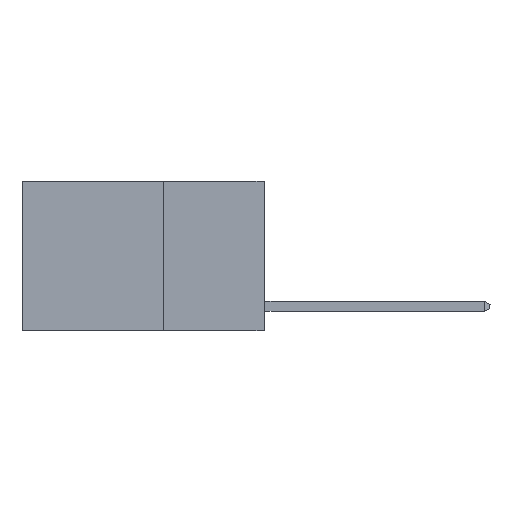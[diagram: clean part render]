
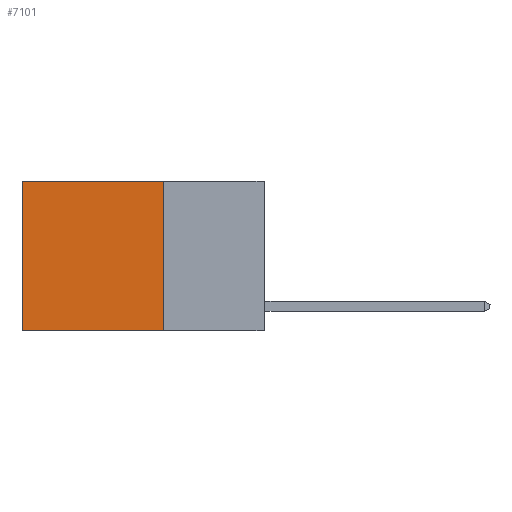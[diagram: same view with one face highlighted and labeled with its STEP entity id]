
A CAD part, left-side view. The second image highlights one B-rep face of the part: STEP entity #7101.
In plain terms, the highlighted planar face has unit normal (-1, 0, 0).
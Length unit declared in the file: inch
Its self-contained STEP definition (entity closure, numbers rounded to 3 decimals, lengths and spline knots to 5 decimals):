
#407 = EDGE_CURVE ( 'NONE', #5967, #1259, #1704, .T. ) ;
#1152 = CARTESIAN_POINT ( 'NONE',  ( 0.2625, 0.25, 0. ) ) ;
#1259 = VERTEX_POINT ( 'NONE', #2028 ) ;
#1391 = AXIS2_PLACEMENT_3D ( 'NONE', #7220, #4628, #16580 ) ;
#1704 = LINE ( 'NONE', #1152, #2133 ) ;
#1827 = ORIENTED_EDGE ( 'NONE', *, *, #407, .F. ) ;
#2028 = CARTESIAN_POINT ( 'NONE',  ( 0.2625, 0.25, -0.37 ) ) ;
#2133 = VECTOR ( 'NONE', #5228, 39.37008 ) ;
#2633 = EDGE_CURVE ( 'NONE', #5967, #14400, #9177, .T. ) ;
#3881 = ORIENTED_EDGE ( 'NONE', *, *, #2633, .T. ) ;
#4152 = VECTOR ( 'NONE', #11414, 39.37008 ) ;
#4333 = CARTESIAN_POINT ( 'NONE',  ( 0.2625, 0.6, 0. ) ) ;
#4628 = DIRECTION ( 'NONE',  ( 1., 0., 0. ) ) ;
#4841 = CARTESIAN_POINT ( 'NONE',  ( 0.2625, 0.25, 0. ) ) ;
#5228 = DIRECTION ( 'NONE',  ( 0., 0., -1. ) ) ;
#5577 = VECTOR ( 'NONE', #14967, 39.37008 ) ;
#5967 = VERTEX_POINT ( 'NONE', #16132 ) ;
#6925 = EDGE_CURVE ( 'NONE', #1259, #7569, #15244, .T. ) ;
#7101 = ADVANCED_FACE ( 'NONE', ( #12118 ), #14595, .F. ) ;
#7220 = CARTESIAN_POINT ( 'NONE',  ( 0.2625, 0.25, 0. ) ) ;
#7569 = VERTEX_POINT ( 'NONE', #11930 ) ;
#7810 = EDGE_LOOP ( 'NONE', ( #15322, #8675, #1827, #3881 ) ) ;
#8675 = ORIENTED_EDGE ( 'NONE', *, *, #6925, .F. ) ;
#9177 = LINE ( 'NONE', #4841, #4152 ) ;
#9689 = CARTESIAN_POINT ( 'NONE',  ( 0.2625, 0.25, -0.37 ) ) ;
#11414 = DIRECTION ( 'NONE',  ( 0., 1., 0. ) ) ;
#11621 = LINE ( 'NONE', #14852, #5577 ) ;
#11930 = CARTESIAN_POINT ( 'NONE',  ( 0.2625, 0.6, -0.37 ) ) ;
#12118 = FACE_OUTER_BOUND ( 'NONE', #7810, .T. ) ;
#13977 = VECTOR ( 'NONE', #17043, 39.37008 ) ;
#14400 = VERTEX_POINT ( 'NONE', #4333 ) ;
#14595 = PLANE ( 'NONE',  #1391 ) ;
#14852 = CARTESIAN_POINT ( 'NONE',  ( 0.2625, 0.6, 0. ) ) ;
#14967 = DIRECTION ( 'NONE',  ( 0., 0., -1. ) ) ;
#15244 = LINE ( 'NONE', #9689, #13977 ) ;
#15322 = ORIENTED_EDGE ( 'NONE', *, *, #15678, .T. ) ;
#15678 = EDGE_CURVE ( 'NONE', #14400, #7569, #11621, .T. ) ;
#16132 = CARTESIAN_POINT ( 'NONE',  ( 0.2625, 0.25, 0. ) ) ;
#16580 = DIRECTION ( 'NONE',  ( 0., 0., -1. ) ) ;
#17043 = DIRECTION ( 'NONE',  ( 0., 1., 0. ) ) ;
